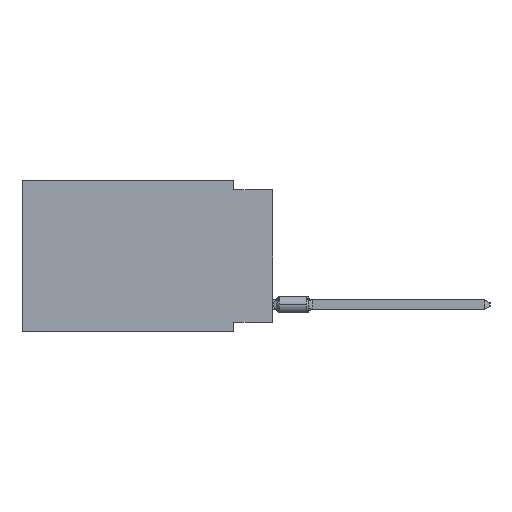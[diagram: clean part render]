
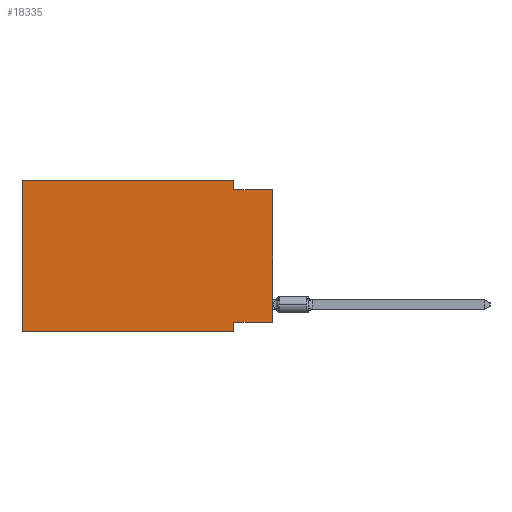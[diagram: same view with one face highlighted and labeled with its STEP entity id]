
A CAD part, left-side view. The second image highlights one B-rep face of the part: STEP entity #18335.
In plain terms, the highlighted planar face has unit normal (-1, 0, 0).
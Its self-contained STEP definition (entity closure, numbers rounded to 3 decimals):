
#72 = LINE ( 'NONE', #9525, #30052 ) ;
#200 = EDGE_CURVE ( 'NONE', #10331, #19395, #21729, .T. ) ;
#304 = CARTESIAN_POINT ( 'NONE',  ( 0., 2.54, -9.906 ) ) ;
#459 = ORIENTED_EDGE ( 'NONE', *, *, #200, .F. ) ;
#1077 = AXIS2_PLACEMENT_3D ( 'NONE', #18609, #9323, #28187 ) ;
#1100 = EDGE_CURVE ( 'NONE', #8221, #14998, #21507, .T. ) ;
#1117 = VERTEX_POINT ( 'NONE', #23986 ) ;
#1349 = VECTOR ( 'NONE', #24279, 1000. ) ;
#1962 = CARTESIAN_POINT ( 'NONE',  ( 0., 16.383, -9.906 ) ) ;
#2198 = CARTESIAN_POINT ( 'NONE',  ( 0., 0., -0.635 ) ) ;
#5005 = CARTESIAN_POINT ( 'NONE',  ( 0., 16.383, 0. ) ) ;
#5841 = VECTOR ( 'NONE', #7509, 1000. ) ;
#6348 = ORIENTED_EDGE ( 'NONE', *, *, #30464, .F. ) ;
#6615 = ORIENTED_EDGE ( 'NONE', *, *, #12290, .T. ) ;
#6710 = VECTOR ( 'NONE', #7295, 1000. ) ;
#7295 = DIRECTION ( 'NONE',  ( 0., 0., 1. ) ) ;
#7509 = DIRECTION ( 'NONE',  ( 0., 0., -1. ) ) ;
#8062 = CARTESIAN_POINT ( 'NONE',  ( 0., 0., -9.271 ) ) ;
#8221 = VERTEX_POINT ( 'NONE', #19200 ) ;
#8413 = VERTEX_POINT ( 'NONE', #15611 ) ;
#9323 = DIRECTION ( 'NONE',  ( 1., 0., 0. ) ) ;
#9525 = CARTESIAN_POINT ( 'NONE',  ( 0., 0., -0.635 ) ) ;
#10331 = VERTEX_POINT ( 'NONE', #17478 ) ;
#10501 = EDGE_CURVE ( 'NONE', #19187, #8413, #10835, .T. ) ;
#10835 = LINE ( 'NONE', #20270, #25922 ) ;
#11998 = DIRECTION ( 'NONE',  ( 0., -1., 0. ) ) ;
#12290 = EDGE_CURVE ( 'NONE', #19187, #14998, #15518, .T. ) ;
#14998 = VERTEX_POINT ( 'NONE', #18342 ) ;
#15518 = LINE ( 'NONE', #15819, #19580 ) ;
#15611 = CARTESIAN_POINT ( 'NONE',  ( 0., 16.383, 0. ) ) ;
#15819 = CARTESIAN_POINT ( 'NONE',  ( 0., 16.383, -9.906 ) ) ;
#16266 = PLANE ( 'NONE',  #1077 ) ;
#16927 = CARTESIAN_POINT ( 'NONE',  ( 0., 2.54, 0. ) ) ;
#17478 = CARTESIAN_POINT ( 'NONE',  ( 0., 2.54, 0. ) ) ;
#18335 = ADVANCED_FACE ( 'NONE', ( #27722 ), #16266, .F. ) ;
#18342 = CARTESIAN_POINT ( 'NONE',  ( 0., 2.54, -9.906 ) ) ;
#18435 = LINE ( 'NONE', #30194, #6710 ) ;
#18609 = CARTESIAN_POINT ( 'NONE',  ( 0., 16.383, 0. ) ) ;
#19187 = VERTEX_POINT ( 'NONE', #1962 ) ;
#19200 = CARTESIAN_POINT ( 'NONE',  ( 0., 2.54, -9.271 ) ) ;
#19248 = DIRECTION ( 'NONE',  ( 0., -1., 0. ) ) ;
#19395 = VERTEX_POINT ( 'NONE', #19907 ) ;
#19580 = VECTOR ( 'NONE', #25265, 1000. ) ;
#19613 = VERTEX_POINT ( 'NONE', #2198 ) ;
#19907 = CARTESIAN_POINT ( 'NONE',  ( 0., 2.54, -0.635 ) ) ;
#20058 = VECTOR ( 'NONE', #23998, 1000. ) ;
#20270 = CARTESIAN_POINT ( 'NONE',  ( 0., 16.383, 0. ) ) ;
#20539 = EDGE_CURVE ( 'NONE', #8413, #10331, #21407, .T. ) ;
#20575 = DIRECTION ( 'NONE',  ( 0., 0., 1. ) ) ;
#21407 = LINE ( 'NONE', #5005, #24938 ) ;
#21507 = LINE ( 'NONE', #304, #1349 ) ;
#21729 = LINE ( 'NONE', #16927, #5841 ) ;
#22449 = EDGE_CURVE ( 'NONE', #19395, #19613, #72, .T. ) ;
#23191 = ORIENTED_EDGE ( 'NONE', *, *, #1100, .F. ) ;
#23986 = CARTESIAN_POINT ( 'NONE',  ( 0., 0., -9.271 ) ) ;
#23998 = DIRECTION ( 'NONE',  ( 0., 1., 0. ) ) ;
#24279 = DIRECTION ( 'NONE',  ( 0., 0., -1. ) ) ;
#24290 = LINE ( 'NONE', #8062, #20058 ) ;
#24938 = VECTOR ( 'NONE', #19248, 1000. ) ;
#25265 = DIRECTION ( 'NONE',  ( 0., -1., 0. ) ) ;
#25755 = ORIENTED_EDGE ( 'NONE', *, *, #30286, .T. ) ;
#25922 = VECTOR ( 'NONE', #20575, 1000. ) ;
#27064 = EDGE_LOOP ( 'NONE', ( #25755, #27149, #459, #27351, #28547, #6615, #23191, #6348 ) ) ;
#27149 = ORIENTED_EDGE ( 'NONE', *, *, #22449, .F. ) ;
#27351 = ORIENTED_EDGE ( 'NONE', *, *, #20539, .F. ) ;
#27722 = FACE_OUTER_BOUND ( 'NONE', #27064, .T. ) ;
#28187 = DIRECTION ( 'NONE',  ( 0., 0., -1. ) ) ;
#28547 = ORIENTED_EDGE ( 'NONE', *, *, #10501, .F. ) ;
#30052 = VECTOR ( 'NONE', #11998, 1000. ) ;
#30194 = CARTESIAN_POINT ( 'NONE',  ( 0., 0., 0. ) ) ;
#30286 = EDGE_CURVE ( 'NONE', #1117, #19613, #18435, .T. ) ;
#30464 = EDGE_CURVE ( 'NONE', #1117, #8221, #24290, .T. ) ;
